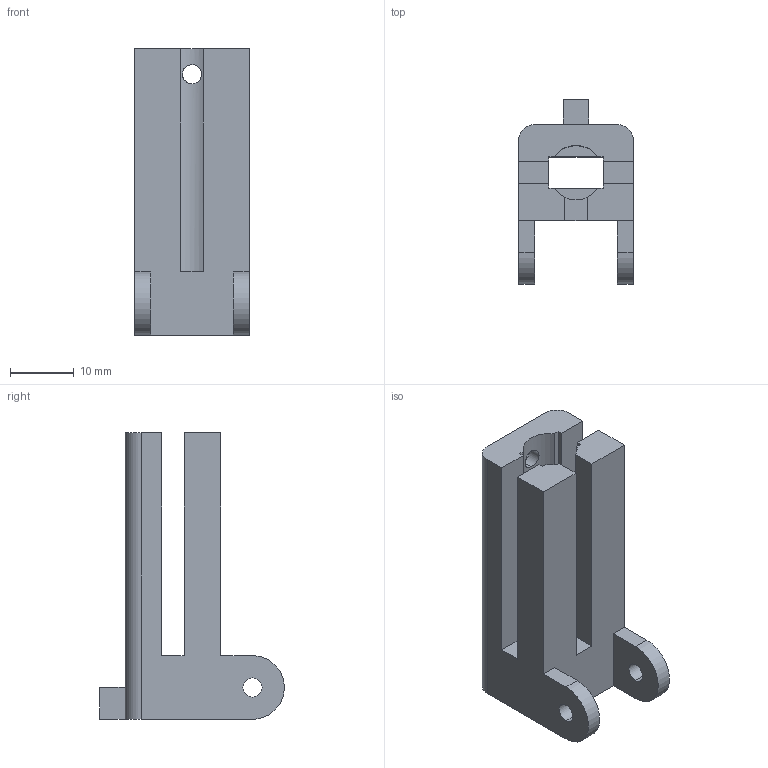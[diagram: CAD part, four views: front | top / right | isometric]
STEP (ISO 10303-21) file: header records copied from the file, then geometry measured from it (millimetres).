
FILE_DESCRIPTION (( 'STEP AP214' ), '1' );
FILE_NAME ('Body_1.STEP', '2014-10-07T00:04:13', ( 'WarFairy' ), ( '' ), 'SwSTEP 2.0', 'SolidWorks 2013', '' );
FILE_SCHEMA (( 'AUTOMOTIVE_DESIGN' ));
Length unit declared in the file: millimetre
Products named in the file (1): Body_1
Bounding box: 18 x 29 x 45 mm (x, y, z)
Volume: 8299 mm3; surface area: 5368 mm2
Topology: 1 solids, 1 shells, 46 faces, 132 edges, 88 vertices
Faces by surface type: plane 32, cylinder 14
Entity records: 1600 total; most frequent: CARTESIAN_POINT 317, ORIENTED_EDGE 264, DIRECTION 252, EDGE_CURVE 132, LINE 102, VECTOR 102, VERTEX_POINT 88, AXIS2_PLACEMENT_3D 75
